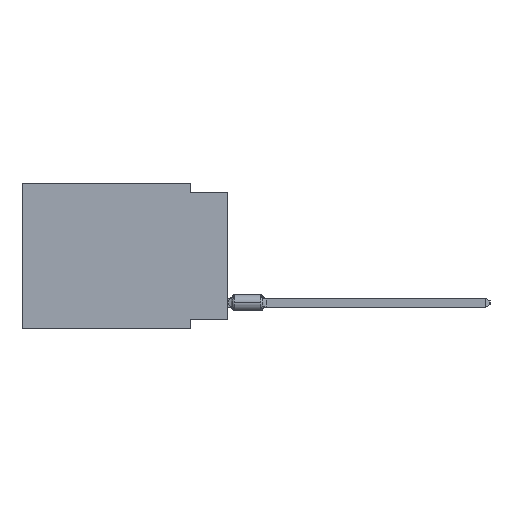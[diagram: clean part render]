
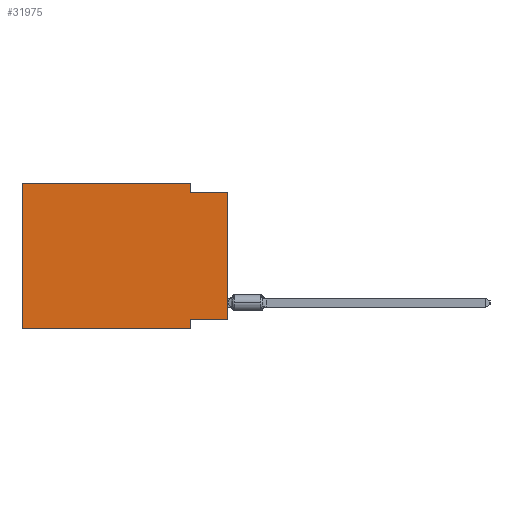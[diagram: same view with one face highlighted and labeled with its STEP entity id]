
A CAD part, left-side view. The second image highlights one B-rep face of the part: STEP entity #31975.
In plain terms, the highlighted planar face has unit normal (-1, 0, 0).
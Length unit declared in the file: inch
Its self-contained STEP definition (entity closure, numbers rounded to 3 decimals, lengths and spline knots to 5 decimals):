
#329 = DIRECTION ( 'NONE',  ( 0., 0., -1. ) ) ;
#640 = VECTOR ( 'NONE', #26790, 39.37008 ) ;
#2145 = VECTOR ( 'NONE', #21445, 39.37008 ) ;
#2648 = CARTESIAN_POINT ( 'NONE',  ( 0., 0.55, 0. ) ) ;
#2820 = PLANE ( 'NONE',  #18825 ) ;
#3032 = CARTESIAN_POINT ( 'NONE',  ( 0., 0.1, 0. ) ) ;
#3066 = EDGE_CURVE ( 'NONE', #19751, #26979, #15016, .T. ) ;
#3282 = ORIENTED_EDGE ( 'NONE', *, *, #19041, .F. ) ;
#3351 = VERTEX_POINT ( 'NONE', #3032 ) ;
#5269 = EDGE_LOOP ( 'NONE', ( #25194, #17150, #29983, #3282, #30007, #31782, #16972, #29293 ) ) ;
#5740 = VECTOR ( 'NONE', #15596, 39.37008 ) ;
#5749 = LINE ( 'NONE', #25960, #5740 ) ;
#5811 = DIRECTION ( 'NONE',  ( 0., -1., 0. ) ) ;
#8292 = DIRECTION ( 'NONE',  ( 1., 0., 0. ) ) ;
#9085 = CARTESIAN_POINT ( 'NONE',  ( 0., 0.55, -0.39 ) ) ;
#10640 = CARTESIAN_POINT ( 'NONE',  ( 0., 0., -0.025 ) ) ;
#10786 = LINE ( 'NONE', #23423, #23244 ) ;
#11040 = EDGE_CURVE ( 'NONE', #19801, #16435, #28564, .T. ) ;
#12657 = DIRECTION ( 'NONE',  ( 0., 0., -1. ) ) ;
#12972 = CARTESIAN_POINT ( 'NONE',  ( 0., 0.55, 0. ) ) ;
#14427 = EDGE_CURVE ( 'NONE', #21283, #19801, #10786, .T. ) ;
#15016 = LINE ( 'NONE', #10640, #24621 ) ;
#15596 = DIRECTION ( 'NONE',  ( 0., -1., 0. ) ) ;
#15941 = DIRECTION ( 'NONE',  ( 0., 0., -1. ) ) ;
#16435 = VERTEX_POINT ( 'NONE', #24507 ) ;
#16908 = LINE ( 'NONE', #31483, #640 ) ;
#16972 = ORIENTED_EDGE ( 'NONE', *, *, #11040, .F. ) ;
#17150 = ORIENTED_EDGE ( 'NONE', *, *, #3066, .F. ) ;
#17454 = CARTESIAN_POINT ( 'NONE',  ( 0., 0.1, 0. ) ) ;
#17807 = EDGE_CURVE ( 'NONE', #24951, #16435, #5749, .T. ) ;
#18056 = VERTEX_POINT ( 'NONE', #2648 ) ;
#18814 = VECTOR ( 'NONE', #329, 39.37008 ) ;
#18825 = AXIS2_PLACEMENT_3D ( 'NONE', #12972, #8292, #12657 ) ;
#18985 = LINE ( 'NONE', #31288, #24899 ) ;
#19041 = EDGE_CURVE ( 'NONE', #18056, #3351, #18985, .T. ) ;
#19751 = VERTEX_POINT ( 'NONE', #25253 ) ;
#19801 = VERTEX_POINT ( 'NONE', #23625 ) ;
#21283 = VERTEX_POINT ( 'NONE', #25937 ) ;
#21445 = DIRECTION ( 'NONE',  ( 0., 0., 1. ) ) ;
#22855 = FACE_OUTER_BOUND ( 'NONE', #5269, .T. ) ;
#23088 = DIRECTION ( 'NONE',  ( 0., 1., 0. ) ) ;
#23136 = EDGE_CURVE ( 'NONE', #3351, #19751, #24581, .T. ) ;
#23244 = VECTOR ( 'NONE', #23088, 39.37008 ) ;
#23423 = CARTESIAN_POINT ( 'NONE',  ( 0., 0., -0.365 ) ) ;
#23625 = CARTESIAN_POINT ( 'NONE',  ( 0., 0.1, -0.365 ) ) ;
#23903 = CARTESIAN_POINT ( 'NONE',  ( 0., 0., -0.025 ) ) ;
#24507 = CARTESIAN_POINT ( 'NONE',  ( 0., 0.1, -0.39 ) ) ;
#24581 = LINE ( 'NONE', #17454, #18814 ) ;
#24621 = VECTOR ( 'NONE', #5811, 39.37008 ) ;
#24899 = VECTOR ( 'NONE', #28869, 39.37008 ) ;
#24951 = VERTEX_POINT ( 'NONE', #9085 ) ;
#25194 = ORIENTED_EDGE ( 'NONE', *, *, #28042, .T. ) ;
#25253 = CARTESIAN_POINT ( 'NONE',  ( 0., 0.1, -0.025 ) ) ;
#25937 = CARTESIAN_POINT ( 'NONE',  ( 0., 0., -0.365 ) ) ;
#25960 = CARTESIAN_POINT ( 'NONE',  ( 0., 0.55, -0.39 ) ) ;
#26460 = CARTESIAN_POINT ( 'NONE',  ( 0., 0., 0. ) ) ;
#26790 = DIRECTION ( 'NONE',  ( 0., 0., 1. ) ) ;
#26979 = VERTEX_POINT ( 'NONE', #23903 ) ;
#27104 = LINE ( 'NONE', #26460, #2145 ) ;
#28042 = EDGE_CURVE ( 'NONE', #21283, #26979, #27104, .T. ) ;
#28564 = LINE ( 'NONE', #31140, #31385 ) ;
#28869 = DIRECTION ( 'NONE',  ( 0., -1., 0. ) ) ;
#29271 = EDGE_CURVE ( 'NONE', #24951, #18056, #16908, .T. ) ;
#29293 = ORIENTED_EDGE ( 'NONE', *, *, #14427, .F. ) ;
#29983 = ORIENTED_EDGE ( 'NONE', *, *, #23136, .F. ) ;
#30007 = ORIENTED_EDGE ( 'NONE', *, *, #29271, .F. ) ;
#31140 = CARTESIAN_POINT ( 'NONE',  ( 0., 0.1, -0.39 ) ) ;
#31288 = CARTESIAN_POINT ( 'NONE',  ( 0., 0.55, 0. ) ) ;
#31385 = VECTOR ( 'NONE', #15941, 39.37008 ) ;
#31483 = CARTESIAN_POINT ( 'NONE',  ( 0., 0.55, 0. ) ) ;
#31782 = ORIENTED_EDGE ( 'NONE', *, *, #17807, .T. ) ;
#31975 = ADVANCED_FACE ( 'NONE', ( #22855 ), #2820, .F. ) ;
